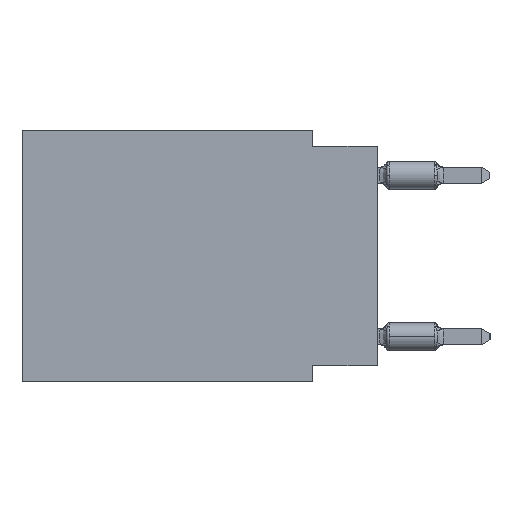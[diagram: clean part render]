
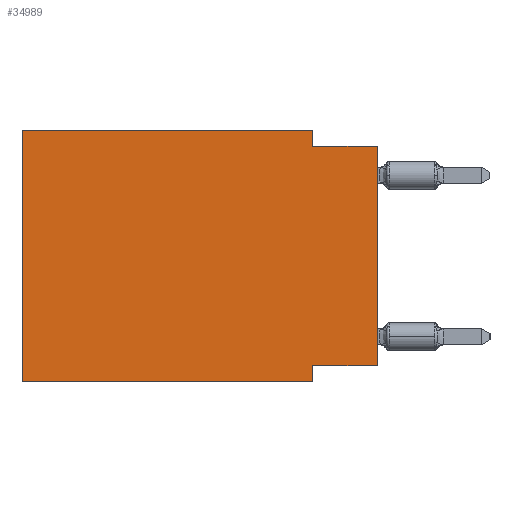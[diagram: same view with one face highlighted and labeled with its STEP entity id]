
A CAD part, left-side view. The second image highlights one B-rep face of the part: STEP entity #34989.
In plain terms, the highlighted planar face has unit normal (-1, 0, 0).
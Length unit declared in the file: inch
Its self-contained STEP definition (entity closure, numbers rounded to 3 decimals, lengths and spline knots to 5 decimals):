
#591 = CARTESIAN_POINT ( 'NONE',  ( 0., 0., -0.365 ) ) ;
#2536 = ORIENTED_EDGE ( 'NONE', *, *, #21574, .F. ) ;
#3078 = LINE ( 'NONE', #38053, #9812 ) ;
#4219 = LINE ( 'NONE', #13440, #32735 ) ;
#4372 = AXIS2_PLACEMENT_3D ( 'NONE', #29895, #36054, #27566 ) ;
#4410 = DIRECTION ( 'NONE',  ( 0., -1., 0. ) ) ;
#4736 = CARTESIAN_POINT ( 'NONE',  ( 0., 0.55, 0. ) ) ;
#4990 = CARTESIAN_POINT ( 'NONE',  ( 0., 0.1, -0.365 ) ) ;
#5351 = ORIENTED_EDGE ( 'NONE', *, *, #23899, .F. ) ;
#6800 = VECTOR ( 'NONE', #10199, 39.37008 ) ;
#7114 = VERTEX_POINT ( 'NONE', #11439 ) ;
#7802 = ORIENTED_EDGE ( 'NONE', *, *, #20689, .F. ) ;
#7872 = ORIENTED_EDGE ( 'NONE', *, *, #16502, .F. ) ;
#8026 = EDGE_LOOP ( 'NONE', ( #12432, #21801, #7802, #5351, #30972, #12573, #7872, #2536 ) ) ;
#9727 = CARTESIAN_POINT ( 'NONE',  ( 0., 0.1, -0.39 ) ) ;
#9812 = VECTOR ( 'NONE', #26640, 39.37008 ) ;
#10199 = DIRECTION ( 'NONE',  ( 0., -1., 0. ) ) ;
#11114 = VERTEX_POINT ( 'NONE', #19501 ) ;
#11439 = CARTESIAN_POINT ( 'NONE',  ( 0., 0.1, -0.025 ) ) ;
#11633 = LINE ( 'NONE', #14540, #25304 ) ;
#12184 = DIRECTION ( 'NONE',  ( 0., 0., 1. ) ) ;
#12432 = ORIENTED_EDGE ( 'NONE', *, *, #15073, .T. ) ;
#12573 = ORIENTED_EDGE ( 'NONE', *, *, #24326, .T. ) ;
#13440 = CARTESIAN_POINT ( 'NONE',  ( 0., 0., -0.025 ) ) ;
#13632 = CARTESIAN_POINT ( 'NONE',  ( 0., 0.55, -0.39 ) ) ;
#14254 = CARTESIAN_POINT ( 'NONE',  ( 0., 0., -0.365 ) ) ;
#14540 = CARTESIAN_POINT ( 'NONE',  ( 0., 0., 0. ) ) ;
#15073 = EDGE_CURVE ( 'NONE', #19222, #11114, #11633, .T. ) ;
#15127 = VERTEX_POINT ( 'NONE', #26349 ) ;
#16502 = EDGE_CURVE ( 'NONE', #33100, #15127, #27337, .T. ) ;
#17200 = VECTOR ( 'NONE', #26060, 39.37008 ) ;
#17377 = EDGE_CURVE ( 'NONE', #22467, #31702, #25945, .T. ) ;
#19222 = VERTEX_POINT ( 'NONE', #591 ) ;
#19501 = CARTESIAN_POINT ( 'NONE',  ( 0., 0., -0.025 ) ) ;
#20689 = EDGE_CURVE ( 'NONE', #25261, #7114, #3078, .T. ) ;
#21574 = EDGE_CURVE ( 'NONE', #19222, #33100, #22762, .T. ) ;
#21801 = ORIENTED_EDGE ( 'NONE', *, *, #24376, .F. ) ;
#22020 = CARTESIAN_POINT ( 'NONE',  ( 0., 0.55, 0. ) ) ;
#22198 = LINE ( 'NONE', #22020, #26551 ) ;
#22349 = LINE ( 'NONE', #13632, #6800 ) ;
#22467 = VERTEX_POINT ( 'NONE', #24152 ) ;
#22762 = LINE ( 'NONE', #14254, #17200 ) ;
#23899 = EDGE_CURVE ( 'NONE', #31702, #25261, #22198, .T. ) ;
#24044 = PLANE ( 'NONE',  #4372 ) ;
#24152 = CARTESIAN_POINT ( 'NONE',  ( 0., 0.55, -0.39 ) ) ;
#24326 = EDGE_CURVE ( 'NONE', #22467, #15127, #22349, .T. ) ;
#24376 = EDGE_CURVE ( 'NONE', #7114, #11114, #4219, .T. ) ;
#24814 = FACE_OUTER_BOUND ( 'NONE', #8026, .T. ) ;
#25261 = VERTEX_POINT ( 'NONE', #32984 ) ;
#25300 = DIRECTION ( 'NONE',  ( 0., -1., 0. ) ) ;
#25304 = VECTOR ( 'NONE', #12184, 39.37008 ) ;
#25945 = LINE ( 'NONE', #26150, #26054 ) ;
#26054 = VECTOR ( 'NONE', #32354, 39.37008 ) ;
#26060 = DIRECTION ( 'NONE',  ( 0., 1., 0. ) ) ;
#26150 = CARTESIAN_POINT ( 'NONE',  ( 0., 0.55, 0. ) ) ;
#26349 = CARTESIAN_POINT ( 'NONE',  ( 0., 0.1, -0.39 ) ) ;
#26551 = VECTOR ( 'NONE', #25300, 39.37008 ) ;
#26640 = DIRECTION ( 'NONE',  ( 0., 0., -1. ) ) ;
#27337 = LINE ( 'NONE', #9727, #37107 ) ;
#27566 = DIRECTION ( 'NONE',  ( 0., 0., -1. ) ) ;
#29895 = CARTESIAN_POINT ( 'NONE',  ( 0., 0.55, 0. ) ) ;
#30972 = ORIENTED_EDGE ( 'NONE', *, *, #17377, .F. ) ;
#31702 = VERTEX_POINT ( 'NONE', #4736 ) ;
#32354 = DIRECTION ( 'NONE',  ( 0., 0., 1. ) ) ;
#32735 = VECTOR ( 'NONE', #4410, 39.37008 ) ;
#32984 = CARTESIAN_POINT ( 'NONE',  ( 0., 0.1, 0. ) ) ;
#33100 = VERTEX_POINT ( 'NONE', #4990 ) ;
#33303 = DIRECTION ( 'NONE',  ( 0., 0., -1. ) ) ;
#34989 = ADVANCED_FACE ( 'NONE', ( #24814 ), #24044, .F. ) ;
#36054 = DIRECTION ( 'NONE',  ( 1., 0., 0. ) ) ;
#37107 = VECTOR ( 'NONE', #33303, 39.37008 ) ;
#38053 = CARTESIAN_POINT ( 'NONE',  ( 0., 0.1, 0. ) ) ;
